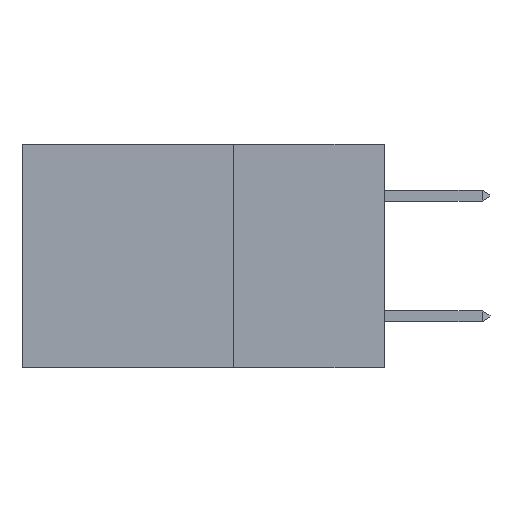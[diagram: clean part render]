
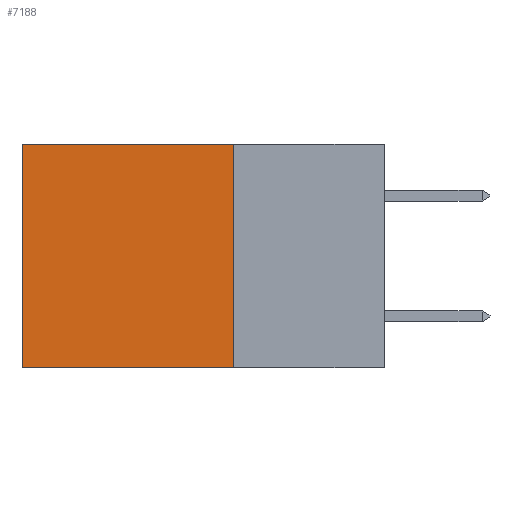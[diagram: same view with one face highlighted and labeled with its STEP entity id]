
A CAD part, left-side view. The second image highlights one B-rep face of the part: STEP entity #7188.
In plain terms, the highlighted planar face has unit normal (-1, 0, 0).
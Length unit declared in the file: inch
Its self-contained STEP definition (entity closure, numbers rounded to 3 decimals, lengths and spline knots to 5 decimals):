
#939 = CARTESIAN_POINT ( 'NONE',  ( 0.2875, 0.6, 0. ) ) ;
#1023 = LINE ( 'NONE', #1983, #4242 ) ;
#1491 = EDGE_CURVE ( 'NONE', #9463, #10336, #7198, .T. ) ;
#1756 = CARTESIAN_POINT ( 'NONE',  ( 0.2875, 0.25, 0. ) ) ;
#1808 = DIRECTION ( 'NONE',  ( 0., 0., -1. ) ) ;
#1983 = CARTESIAN_POINT ( 'NONE',  ( 0.2875, 0.25, -0.37 ) ) ;
#2017 = DIRECTION ( 'NONE',  ( 1., 0., 0. ) ) ;
#2287 = VERTEX_POINT ( 'NONE', #11123 ) ;
#2501 = ORIENTED_EDGE ( 'NONE', *, *, #9805, .T. ) ;
#2899 = FACE_OUTER_BOUND ( 'NONE', #8392, .T. ) ;
#3018 = CARTESIAN_POINT ( 'NONE',  ( 0.2875, 0.25, 0. ) ) ;
#3192 = LINE ( 'NONE', #3018, #4965 ) ;
#3496 = CARTESIAN_POINT ( 'NONE',  ( 0.2875, 0.25, -0.37 ) ) ;
#4054 = VECTOR ( 'NONE', #6165, 39.37008 ) ;
#4066 = CARTESIAN_POINT ( 'NONE',  ( 0.2875, 0.6, -0.37 ) ) ;
#4242 = VECTOR ( 'NONE', #9775, 39.37008 ) ;
#4679 = CARTESIAN_POINT ( 'NONE',  ( 0.2875, 0.6, 0. ) ) ;
#4965 = VECTOR ( 'NONE', #8297, 39.37008 ) ;
#5001 = ORIENTED_EDGE ( 'NONE', *, *, #1491, .T. ) ;
#6165 = DIRECTION ( 'NONE',  ( 0., 0., -1. ) ) ;
#6211 = VERTEX_POINT ( 'NONE', #3496 ) ;
#6252 = EDGE_CURVE ( 'NONE', #6211, #10336, #1023, .T. ) ;
#6973 = ORIENTED_EDGE ( 'NONE', *, *, #6252, .F. ) ;
#7085 = PLANE ( 'NONE',  #10994 ) ;
#7188 = ADVANCED_FACE ( 'NONE', ( #2899 ), #7085, .F. ) ;
#7198 = LINE ( 'NONE', #939, #4054 ) ;
#7203 = CARTESIAN_POINT ( 'NONE',  ( 0.2875, 0.25, 0. ) ) ;
#7668 = ORIENTED_EDGE ( 'NONE', *, *, #11027, .F. ) ;
#8119 = DIRECTION ( 'NONE',  ( 0., 0., -1. ) ) ;
#8297 = DIRECTION ( 'NONE',  ( 0., 1., 0. ) ) ;
#8392 = EDGE_LOOP ( 'NONE', ( #5001, #6973, #7668, #2501 ) ) ;
#8903 = VECTOR ( 'NONE', #1808, 39.37008 ) ;
#9463 = VERTEX_POINT ( 'NONE', #4679 ) ;
#9775 = DIRECTION ( 'NONE',  ( 0., 1., 0. ) ) ;
#9805 = EDGE_CURVE ( 'NONE', #2287, #9463, #3192, .T. ) ;
#10336 = VERTEX_POINT ( 'NONE', #4066 ) ;
#10994 = AXIS2_PLACEMENT_3D ( 'NONE', #7203, #2017, #8119 ) ;
#11027 = EDGE_CURVE ( 'NONE', #2287, #6211, #11290, .T. ) ;
#11123 = CARTESIAN_POINT ( 'NONE',  ( 0.2875, 0.25, 0. ) ) ;
#11290 = LINE ( 'NONE', #1756, #8903 ) ;
